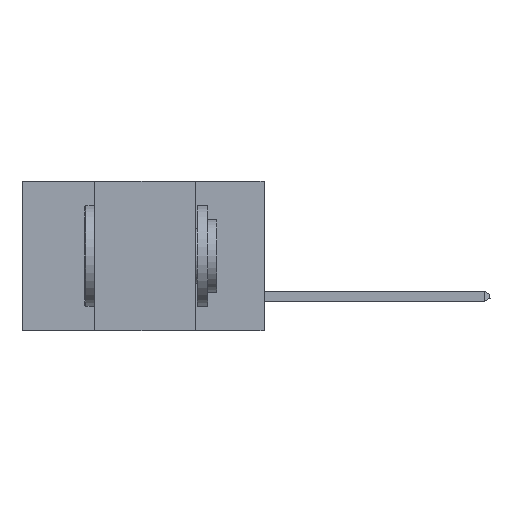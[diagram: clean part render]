
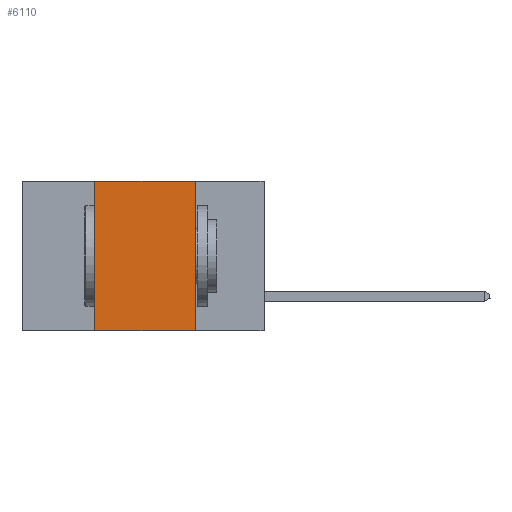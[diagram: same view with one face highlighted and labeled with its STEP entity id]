
A CAD part, left-side view. The second image highlights one B-rep face of the part: STEP entity #6110.
In plain terms, the highlighted planar face has unit normal (-1, 0, 0).
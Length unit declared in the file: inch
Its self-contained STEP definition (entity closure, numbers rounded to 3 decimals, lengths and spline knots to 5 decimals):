
#35 = FACE_OUTER_BOUND ( 'NONE', #483, .T. ) ;
#232 = CARTESIAN_POINT ( 'NONE',  ( 0., 0.6, 0. ) ) ;
#405 = DIRECTION ( 'NONE',  ( 0., 0., 1. ) ) ;
#483 = EDGE_LOOP ( 'NONE', ( #6872, #7120, #6729, #5411 ) ) ;
#493 = EDGE_CURVE ( 'NONE', #11061, #2290, #10893, .T. ) ;
#1820 = EDGE_CURVE ( 'NONE', #2262, #4554, #7977, .T. ) ;
#1847 = PLANE ( 'NONE',  #9949 ) ;
#1923 = VECTOR ( 'NONE', #7124, 39.37008 ) ;
#2084 = CARTESIAN_POINT ( 'NONE',  ( 0., 0.42, -0.37 ) ) ;
#2086 = LINE ( 'NONE', #8712, #6442 ) ;
#2262 = VERTEX_POINT ( 'NONE', #8430 ) ;
#2290 = VERTEX_POINT ( 'NONE', #4915 ) ;
#2611 = EDGE_CURVE ( 'NONE', #11061, #4554, #2086, .T. ) ;
#3275 = LINE ( 'NONE', #232, #1923 ) ;
#3544 = DIRECTION ( 'NONE',  ( 0., -1., 0. ) ) ;
#4021 = VECTOR ( 'NONE', #405, 39.37008 ) ;
#4554 = VERTEX_POINT ( 'NONE', #7644 ) ;
#4915 = CARTESIAN_POINT ( 'NONE',  ( 0., 0.42, 0. ) ) ;
#5266 = DIRECTION ( 'NONE',  ( 0., 0., -1. ) ) ;
#5411 = ORIENTED_EDGE ( 'NONE', *, *, #2611, .T. ) ;
#6110 = ADVANCED_FACE ( 'NONE', ( #35 ), #1847, .F. ) ;
#6168 = DIRECTION ( 'NONE',  ( 1., 0., 0. ) ) ;
#6442 = VECTOR ( 'NONE', #3544, 39.37008 ) ;
#6729 = ORIENTED_EDGE ( 'NONE', *, *, #493, .F. ) ;
#6872 = ORIENTED_EDGE ( 'NONE', *, *, #1820, .F. ) ;
#7120 = ORIENTED_EDGE ( 'NONE', *, *, #10868, .F. ) ;
#7124 = DIRECTION ( 'NONE',  ( 0., -1., 0. ) ) ;
#7644 = CARTESIAN_POINT ( 'NONE',  ( 0., 0.17, -0.37 ) ) ;
#7868 = CARTESIAN_POINT ( 'NONE',  ( 0., 0.17, 0. ) ) ;
#7977 = LINE ( 'NONE', #7868, #11082 ) ;
#8430 = CARTESIAN_POINT ( 'NONE',  ( 0., 0.17, 0. ) ) ;
#8712 = CARTESIAN_POINT ( 'NONE',  ( 0., 0.6, -0.37 ) ) ;
#9505 = DIRECTION ( 'NONE',  ( 0., 0., -1. ) ) ;
#9714 = CARTESIAN_POINT ( 'NONE',  ( 0., 0.6, 0. ) ) ;
#9949 = AXIS2_PLACEMENT_3D ( 'NONE', #9714, #6168, #5266 ) ;
#10594 = CARTESIAN_POINT ( 'NONE',  ( 0., 0.42, 0. ) ) ;
#10868 = EDGE_CURVE ( 'NONE', #2290, #2262, #3275, .T. ) ;
#10893 = LINE ( 'NONE', #10594, #4021 ) ;
#11061 = VERTEX_POINT ( 'NONE', #2084 ) ;
#11082 = VECTOR ( 'NONE', #9505, 39.37008 ) ;
